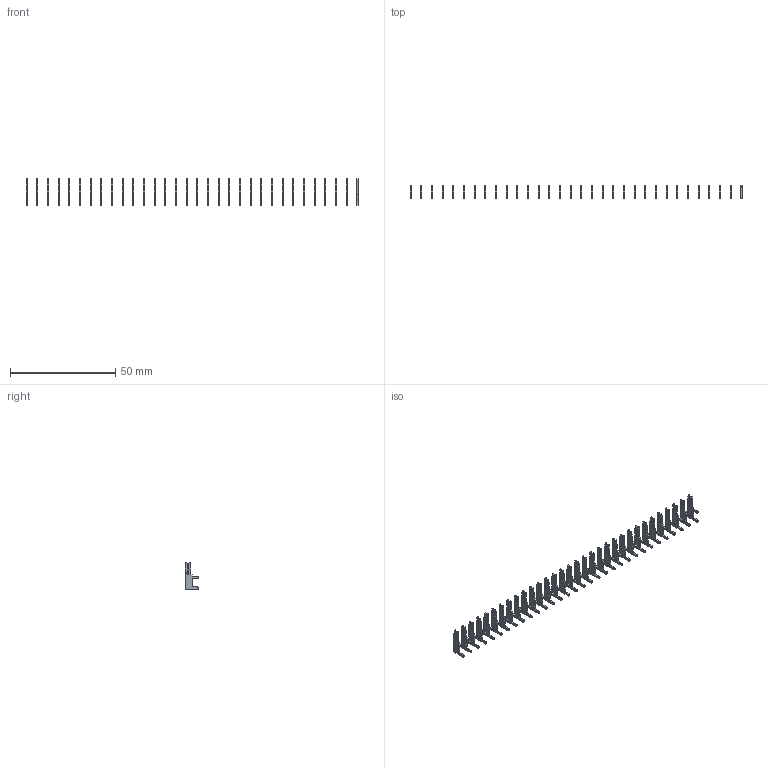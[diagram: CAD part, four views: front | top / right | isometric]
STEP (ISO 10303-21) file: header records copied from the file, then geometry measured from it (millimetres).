
FILE_DESCRIPTION (( 'STEP AP203' ), '1' );
FILE_NAME ('105-032-203-200.STEP', '2020-08-29T23:41:35', ( '' ), ( '' ), 'SwSTEP 2.0', 'SolidWorks 2020', '' );
FILE_SCHEMA (( 'CONFIG_CONTROL_DESIGN' ));
Length unit declared in the file: inch
Products named in the file (2): 105-032-203-200; 100-290-001_100-290-203
Assembly tree (32 placements, depth 2):
  105-032-203-200
    100-290-001_100-290-203  x32
Bounding box: 158.08 x 6.53 x 12.7 mm (x, y, z)
Volume: 807.9 mm3; surface area: 3703 mm2
Topology: 32 solids, 32 shells, 896 faces, 2496 edges, 1664 vertices
Faces by surface type: plane 672, cylinder 224
Entity records: 2088 total; most frequent: DIRECTION 214, CARTESIAN_POINT 205, ORIENTED_EDGE 156, EDGE_CURVE 78, AXIS2_PLACEMENT_3D 77, LOCAL_TIME 74, DATE_AND_TIME 74, COORDINATED_UNIVERSAL_TIME_OFFSET 74
